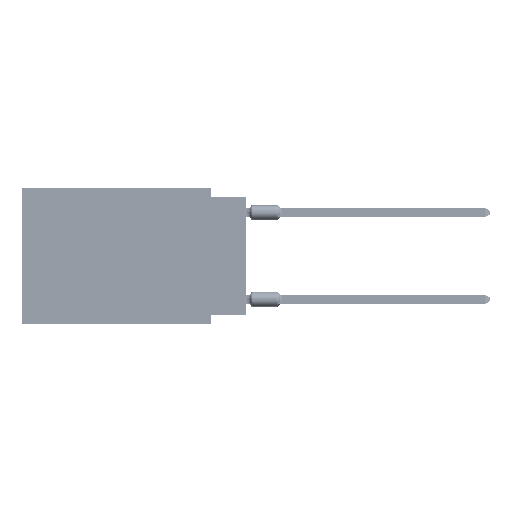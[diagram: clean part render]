
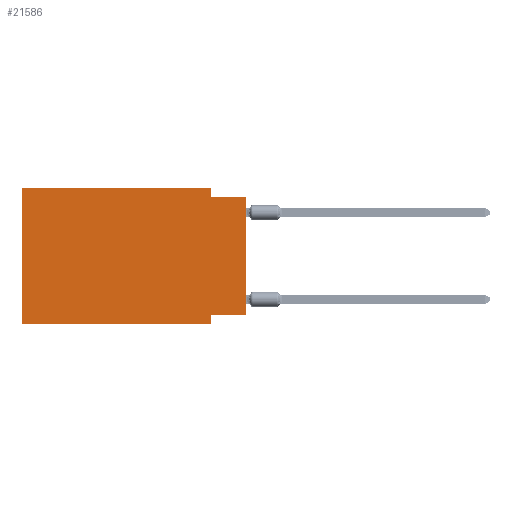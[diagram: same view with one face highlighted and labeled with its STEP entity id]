
A CAD part, left-side view. The second image highlights one B-rep face of the part: STEP entity #21586.
In plain terms, the highlighted planar face has unit normal (-1, 0, 0).
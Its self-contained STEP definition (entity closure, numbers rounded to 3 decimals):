
#686 = CARTESIAN_POINT ( 'NONE',  ( 0., 0., -9.271 ) ) ;
#3477 = ORIENTED_EDGE ( 'NONE', *, *, #44698, .F. ) ;
#4441 = AXIS2_PLACEMENT_3D ( 'NONE', #68094, #38463, #74989 ) ;
#6832 = CARTESIAN_POINT ( 'NONE',  ( 0., 2.54, -9.271 ) ) ;
#8261 = CARTESIAN_POINT ( 'NONE',  ( 0., 2.54, -9.906 ) ) ;
#10444 = CARTESIAN_POINT ( 'NONE',  ( 0., 0., -9.271 ) ) ;
#13684 = PLANE ( 'NONE',  #4441 ) ;
#14326 = VERTEX_POINT ( 'NONE', #39329 ) ;
#16112 = DIRECTION ( 'NONE',  ( 0., 0., 1. ) ) ;
#16433 = CARTESIAN_POINT ( 'NONE',  ( 0., 16.383, 0. ) ) ;
#16666 = CARTESIAN_POINT ( 'NONE',  ( 0., 16.383, -9.906 ) ) ;
#20564 = DIRECTION ( 'NONE',  ( 0., 1., 0. ) ) ;
#21099 = VECTOR ( 'NONE', #20564, 1000. ) ;
#21586 = ADVANCED_FACE ( 'NONE', ( #50234 ), #13684, .F. ) ;
#24811 = CARTESIAN_POINT ( 'NONE',  ( 0., 0., -0.635 ) ) ;
#26640 = VECTOR ( 'NONE', #68234, 1000. ) ;
#29021 = DIRECTION ( 'NONE',  ( 0., 0., 1. ) ) ;
#30588 = EDGE_CURVE ( 'NONE', #48370, #37421, #50615, .T. ) ;
#32292 = CARTESIAN_POINT ( 'NONE',  ( 0., 2.54, 0. ) ) ;
#33220 = CARTESIAN_POINT ( 'NONE',  ( 0., 16.383, 0. ) ) ;
#34491 = ORIENTED_EDGE ( 'NONE', *, *, #63565, .F. ) ;
#36542 = DIRECTION ( 'NONE',  ( 0., -1., 0. ) ) ;
#37421 = VERTEX_POINT ( 'NONE', #6832 ) ;
#38463 = DIRECTION ( 'NONE',  ( 1., 0., 0. ) ) ;
#38689 = VECTOR ( 'NONE', #36542, 1000. ) ;
#39329 = CARTESIAN_POINT ( 'NONE',  ( 0., 16.383, 0. ) ) ;
#40074 = CARTESIAN_POINT ( 'NONE',  ( 0., 0., -0.635 ) ) ;
#40961 = VECTOR ( 'NONE', #29021, 1000. ) ;
#41917 = ORIENTED_EDGE ( 'NONE', *, *, #62670, .F. ) ;
#43767 = ORIENTED_EDGE ( 'NONE', *, *, #77677, .T. ) ;
#44698 = EDGE_CURVE ( 'NONE', #60664, #49468, #69034, .T. ) ;
#44996 = CARTESIAN_POINT ( 'NONE',  ( 0., 2.54, 0. ) ) ;
#47306 = CARTESIAN_POINT ( 'NONE',  ( 0., 2.54, -9.906 ) ) ;
#48370 = VERTEX_POINT ( 'NONE', #10444 ) ;
#49468 = VERTEX_POINT ( 'NONE', #40074 ) ;
#50234 = FACE_OUTER_BOUND ( 'NONE', #68842, .T. ) ;
#50615 = LINE ( 'NONE', #686, #21099 ) ;
#51971 = EDGE_CURVE ( 'NONE', #48370, #49468, #71334, .T. ) ;
#57984 = DIRECTION ( 'NONE',  ( 0., -1., 0. ) ) ;
#60100 = LINE ( 'NONE', #16666, #38689 ) ;
#60664 = VERTEX_POINT ( 'NONE', #71115 ) ;
#61843 = VERTEX_POINT ( 'NONE', #32292 ) ;
#62615 = EDGE_CURVE ( 'NONE', #61843, #60664, #68944, .T. ) ;
#62662 = LINE ( 'NONE', #8261, #75372 ) ;
#62670 = EDGE_CURVE ( 'NONE', #14326, #61843, #70142, .T. ) ;
#63565 = EDGE_CURVE ( 'NONE', #37421, #77315, #62662, .T. ) ;
#66047 = CARTESIAN_POINT ( 'NONE',  ( 0., 0., 0. ) ) ;
#66356 = LINE ( 'NONE', #16433, #40961 ) ;
#67495 = VECTOR ( 'NONE', #57984, 1000. ) ;
#68025 = ORIENTED_EDGE ( 'NONE', *, *, #51971, .T. ) ;
#68094 = CARTESIAN_POINT ( 'NONE',  ( 0., 16.383, 0. ) ) ;
#68234 = DIRECTION ( 'NONE',  ( 0., -1., 0. ) ) ;
#68842 = EDGE_LOOP ( 'NONE', ( #68025, #3477, #76531, #41917, #74022, #43767, #34491, #70511 ) ) ;
#68944 = LINE ( 'NONE', #44996, #75257 ) ;
#69034 = LINE ( 'NONE', #24811, #26640 ) ;
#69552 = DIRECTION ( 'NONE',  ( 0., 0., -1. ) ) ;
#70142 = LINE ( 'NONE', #33220, #67495 ) ;
#70511 = ORIENTED_EDGE ( 'NONE', *, *, #30588, .F. ) ;
#71115 = CARTESIAN_POINT ( 'NONE',  ( 0., 2.54, -0.635 ) ) ;
#71334 = LINE ( 'NONE', #66047, #75316 ) ;
#72812 = EDGE_CURVE ( 'NONE', #75531, #14326, #66356, .T. ) ;
#74022 = ORIENTED_EDGE ( 'NONE', *, *, #72812, .F. ) ;
#74989 = DIRECTION ( 'NONE',  ( 0., 0., -1. ) ) ;
#75038 = DIRECTION ( 'NONE',  ( 0., 0., -1. ) ) ;
#75257 = VECTOR ( 'NONE', #75038, 1000. ) ;
#75316 = VECTOR ( 'NONE', #16112, 1000. ) ;
#75372 = VECTOR ( 'NONE', #69552, 1000. ) ;
#75531 = VERTEX_POINT ( 'NONE', #79749 ) ;
#76531 = ORIENTED_EDGE ( 'NONE', *, *, #62615, .F. ) ;
#77315 = VERTEX_POINT ( 'NONE', #47306 ) ;
#77677 = EDGE_CURVE ( 'NONE', #75531, #77315, #60100, .T. ) ;
#79749 = CARTESIAN_POINT ( 'NONE',  ( 0., 16.383, -9.906 ) ) ;
